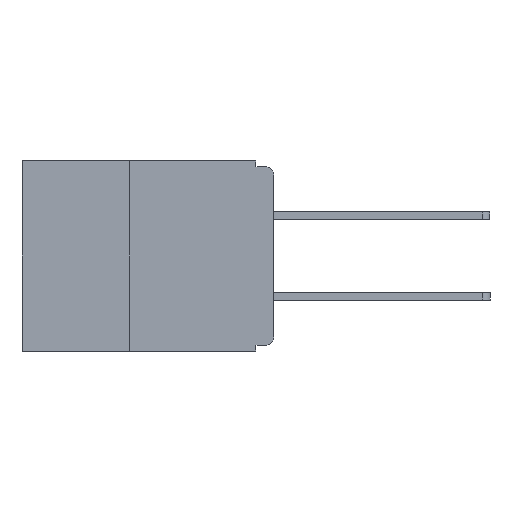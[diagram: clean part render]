
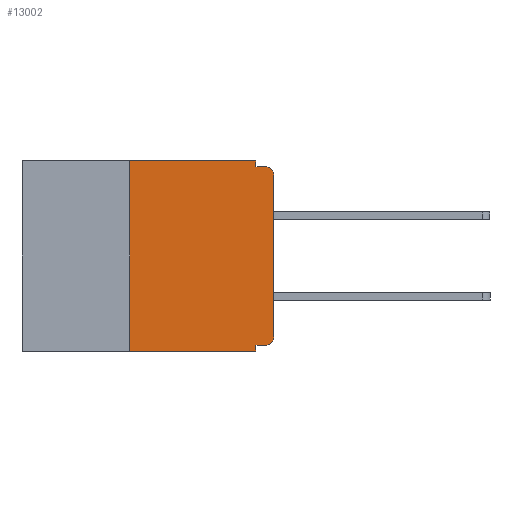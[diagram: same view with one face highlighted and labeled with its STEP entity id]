
A CAD part, left-side view. The second image highlights one B-rep face of the part: STEP entity #13002.
In plain terms, the highlighted planar face has unit normal (-1, 0, 0).
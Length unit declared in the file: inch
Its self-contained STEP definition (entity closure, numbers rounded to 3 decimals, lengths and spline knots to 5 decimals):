
#544 = LINE ( 'NONE', #15795, #20144 ) ;
#594 = CARTESIAN_POINT ( 'NONE',  ( 0., 0.25, 0. ) ) ;
#598 = DIRECTION ( 'NONE',  ( 0., 0., -1. ) ) ;
#643 = DIRECTION ( 'NONE',  ( -1., 0., 0. ) ) ;
#648 = CARTESIAN_POINT ( 'NONE',  ( 0., 0.015, -0.305 ) ) ;
#1549 = CARTESIAN_POINT ( 'NONE',  ( 0., 0.031, 0. ) ) ;
#2451 = VECTOR ( 'NONE', #10794, 39.37008 ) ;
#2846 = VERTEX_POINT ( 'NONE', #15236 ) ;
#3027 = CARTESIAN_POINT ( 'NONE',  ( 0., 0.437, 0. ) ) ;
#3247 = VECTOR ( 'NONE', #21644, 39.37008 ) ;
#3393 = EDGE_CURVE ( 'NONE', #5733, #19156, #4137, .T. ) ;
#4044 = EDGE_CURVE ( 'NONE', #17828, #21724, #14953, .T. ) ;
#4137 = LINE ( 'NONE', #4836, #10534 ) ;
#4180 = VERTEX_POINT ( 'NONE', #23683 ) ;
#4468 = LINE ( 'NONE', #7961, #9088 ) ;
#4487 = DIRECTION ( 'NONE',  ( -1., 0., 0. ) ) ;
#4836 = CARTESIAN_POINT ( 'NONE',  ( 0., 0., 0. ) ) ;
#4900 = DIRECTION ( 'NONE',  ( 0., 0., 1. ) ) ;
#5066 = DIRECTION ( 'NONE',  ( 0., 0., -1. ) ) ;
#5253 = EDGE_CURVE ( 'NONE', #2846, #5733, #24167, .T. ) ;
#5411 = EDGE_CURVE ( 'NONE', #4180, #21724, #20836, .T. ) ;
#5733 = VERTEX_POINT ( 'NONE', #7810 ) ;
#6119 = CARTESIAN_POINT ( 'NONE',  ( 0., 0.015, -0.01 ) ) ;
#6160 = VERTEX_POINT ( 'NONE', #20894 ) ;
#6419 = DIRECTION ( 'NONE',  ( 0., 0., -1. ) ) ;
#6786 = EDGE_CURVE ( 'NONE', #4180, #15458, #12754, .T. ) ;
#7430 = CIRCLE ( 'NONE', #7460, 0.015 ) ;
#7460 = AXIS2_PLACEMENT_3D ( 'NONE', #15905, #4487, #17747 ) ;
#7810 = CARTESIAN_POINT ( 'NONE',  ( 0., 0., -0.305 ) ) ;
#7932 = EDGE_CURVE ( 'NONE', #19156, #10243, #7430, .T. ) ;
#7961 = CARTESIAN_POINT ( 'NONE',  ( 0., 0.437, 0. ) ) ;
#8506 = EDGE_LOOP ( 'NONE', ( #11822, #12384, #15463, #16345, #16673, #17953, #18327, #18523, #19413, #19875 ) ) ;
#8667 = AXIS2_PLACEMENT_3D ( 'NONE', #648, #643, #598 ) ;
#8919 = PLANE ( 'NONE',  #22933 ) ;
#9088 = VECTOR ( 'NONE', #19063, 39.37008 ) ;
#9314 = EDGE_CURVE ( 'NONE', #15640, #6160, #10435, .T. ) ;
#9569 = CARTESIAN_POINT ( 'NONE',  ( 0., 0.031, -0.33 ) ) ;
#9939 = VECTOR ( 'NONE', #6419, 39.37008 ) ;
#10044 = CARTESIAN_POINT ( 'NONE',  ( 0., 0., -0.025 ) ) ;
#10243 = VERTEX_POINT ( 'NONE', #6119 ) ;
#10435 = LINE ( 'NONE', #23938, #15425 ) ;
#10534 = VECTOR ( 'NONE', #4900, 39.37008 ) ;
#10794 = DIRECTION ( 'NONE',  ( 0., 0., 1. ) ) ;
#10852 = CARTESIAN_POINT ( 'NONE',  ( 0., 0.25, -0.33 ) ) ;
#11044 = VECTOR ( 'NONE', #18242, 39.37008 ) ;
#11345 = CARTESIAN_POINT ( 'NONE',  ( 0., 0.031, -0.33 ) ) ;
#11822 = ORIENTED_EDGE ( 'NONE', *, *, #3393, .T. ) ;
#12135 = DIRECTION ( 'NONE',  ( 0., -1., 0. ) ) ;
#12384 = ORIENTED_EDGE ( 'NONE', *, *, #7932, .T. ) ;
#12689 = EDGE_CURVE ( 'NONE', #15458, #15640, #4468, .T. ) ;
#12754 = LINE ( 'NONE', #10852, #2451 ) ;
#12938 = EDGE_CURVE ( 'NONE', #2846, #17828, #13526, .T. ) ;
#13002 = ADVANCED_FACE ( 'NONE', ( #17270 ), #8919, .F. ) ;
#13526 = LINE ( 'NONE', #19818, #3247 ) ;
#14953 = LINE ( 'NONE', #9569, #9939 ) ;
#15236 = CARTESIAN_POINT ( 'NONE',  ( 0., 0.015, -0.32 ) ) ;
#15425 = VECTOR ( 'NONE', #20354, 39.37008 ) ;
#15458 = VERTEX_POINT ( 'NONE', #594 ) ;
#15463 = ORIENTED_EDGE ( 'NONE', *, *, #20290, .F. ) ;
#15640 = VERTEX_POINT ( 'NONE', #1549 ) ;
#15795 = CARTESIAN_POINT ( 'NONE',  ( 0., 0., -0.01 ) ) ;
#15905 = CARTESIAN_POINT ( 'NONE',  ( 0., 0.015, -0.025 ) ) ;
#16345 = ORIENTED_EDGE ( 'NONE', *, *, #9314, .F. ) ;
#16401 = DIRECTION ( 'NONE',  ( 1., 0., 0. ) ) ;
#16673 = ORIENTED_EDGE ( 'NONE', *, *, #12689, .F. ) ;
#17270 = FACE_OUTER_BOUND ( 'NONE', #8506, .T. ) ;
#17747 = DIRECTION ( 'NONE',  ( 0., 0., -1. ) ) ;
#17828 = VERTEX_POINT ( 'NONE', #18646 ) ;
#17953 = ORIENTED_EDGE ( 'NONE', *, *, #6786, .F. ) ;
#18165 = CARTESIAN_POINT ( 'NONE',  ( 0., 0.437, -0.33 ) ) ;
#18242 = DIRECTION ( 'NONE',  ( 0., -1., 0. ) ) ;
#18327 = ORIENTED_EDGE ( 'NONE', *, *, #5411, .T. ) ;
#18523 = ORIENTED_EDGE ( 'NONE', *, *, #4044, .F. ) ;
#18646 = CARTESIAN_POINT ( 'NONE',  ( 0., 0.031, -0.32 ) ) ;
#19063 = DIRECTION ( 'NONE',  ( 0., -1., 0. ) ) ;
#19156 = VERTEX_POINT ( 'NONE', #10044 ) ;
#19413 = ORIENTED_EDGE ( 'NONE', *, *, #12938, .F. ) ;
#19818 = CARTESIAN_POINT ( 'NONE',  ( 0., 0., -0.32 ) ) ;
#19875 = ORIENTED_EDGE ( 'NONE', *, *, #5253, .T. ) ;
#20144 = VECTOR ( 'NONE', #12135, 39.37008 ) ;
#20290 = EDGE_CURVE ( 'NONE', #6160, #10243, #544, .T. ) ;
#20354 = DIRECTION ( 'NONE',  ( 0., 0., -1. ) ) ;
#20836 = LINE ( 'NONE', #18165, #11044 ) ;
#20894 = CARTESIAN_POINT ( 'NONE',  ( 0., 0.031, -0.01 ) ) ;
#21644 = DIRECTION ( 'NONE',  ( 0., 1., 0. ) ) ;
#21724 = VERTEX_POINT ( 'NONE', #11345 ) ;
#22933 = AXIS2_PLACEMENT_3D ( 'NONE', #3027, #16401, #5066 ) ;
#23683 = CARTESIAN_POINT ( 'NONE',  ( 0., 0.25, -0.33 ) ) ;
#23938 = CARTESIAN_POINT ( 'NONE',  ( 0., 0.031, 0. ) ) ;
#24167 = CIRCLE ( 'NONE', #8667, 0.015 ) ;
